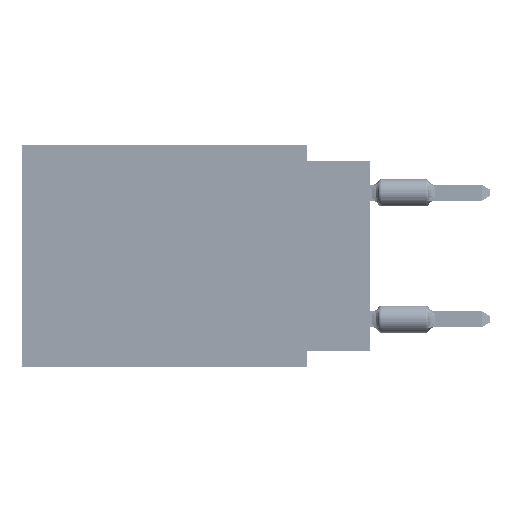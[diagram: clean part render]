
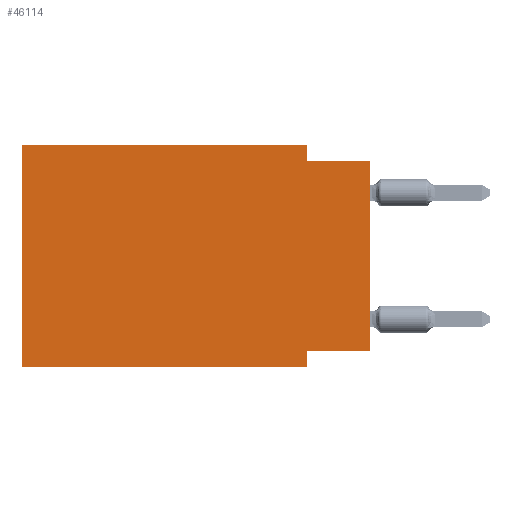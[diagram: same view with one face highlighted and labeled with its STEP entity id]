
A CAD part, left-side view. The second image highlights one B-rep face of the part: STEP entity #46114.
In plain terms, the highlighted planar face has unit normal (-1, 0, 0).
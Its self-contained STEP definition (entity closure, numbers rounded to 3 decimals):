
#430 = VECTOR ( 'NONE', #18082, 1000. ) ;
#1120 = VERTEX_POINT ( 'NONE', #33588 ) ;
#1628 = CARTESIAN_POINT ( 'NONE',  ( 0., 2.54, -8.255 ) ) ;
#1795 = DIRECTION ( 'NONE',  ( 0., 0., 1. ) ) ;
#2242 = VECTOR ( 'NONE', #56492, 1000. ) ;
#2879 = LINE ( 'NONE', #26406, #430 ) ;
#7391 = CARTESIAN_POINT ( 'NONE',  ( 0., 13.97, 0. ) ) ;
#7825 = VECTOR ( 'NONE', #49756, 1000. ) ;
#9047 = EDGE_CURVE ( 'NONE', #80433, #78331, #52441, .T. ) ;
#10928 = CARTESIAN_POINT ( 'NONE',  ( 0., 2.54, -0.635 ) ) ;
#13203 = VECTOR ( 'NONE', #89254, 1000. ) ;
#13825 = ORIENTED_EDGE ( 'NONE', *, *, #69051, .T. ) ;
#15236 = DIRECTION ( 'NONE',  ( 0., 0., 1. ) ) ;
#16129 = EDGE_CURVE ( 'NONE', #66606, #78331, #87042, .T. ) ;
#16884 = ORIENTED_EDGE ( 'NONE', *, *, #49032, .F. ) ;
#18082 = DIRECTION ( 'NONE',  ( 0., 0., -1. ) ) ;
#19843 = CARTESIAN_POINT ( 'NONE',  ( 0., 13.97, -8.89 ) ) ;
#21167 = CARTESIAN_POINT ( 'NONE',  ( 0., 13.97, 0. ) ) ;
#21896 = CARTESIAN_POINT ( 'NONE',  ( 0., 2.54, -8.89 ) ) ;
#23350 = EDGE_CURVE ( 'NONE', #74898, #35920, #65322, .T. ) ;
#25689 = EDGE_CURVE ( 'NONE', #66606, #74898, #52506, .T. ) ;
#26406 = CARTESIAN_POINT ( 'NONE',  ( 0., 2.54, 0. ) ) ;
#28214 = CARTESIAN_POINT ( 'NONE',  ( 0., 13.97, 0. ) ) ;
#28435 = VECTOR ( 'NONE', #1795, 1000. ) ;
#30696 = VECTOR ( 'NONE', #52971, 1000. ) ;
#33588 = CARTESIAN_POINT ( 'NONE',  ( 0., 0., -0.635 ) ) ;
#35566 = FACE_OUTER_BOUND ( 'NONE', #51093, .T. ) ;
#35920 = VERTEX_POINT ( 'NONE', #42188 ) ;
#36294 = CARTESIAN_POINT ( 'NONE',  ( 0., 13.97, 0. ) ) ;
#37706 = CARTESIAN_POINT ( 'NONE',  ( 0., 0., -8.255 ) ) ;
#38013 = AXIS2_PLACEMENT_3D ( 'NONE', #28214, #58125, #72854 ) ;
#39083 = CARTESIAN_POINT ( 'NONE',  ( 0., 0., 0. ) ) ;
#41335 = EDGE_CURVE ( 'NONE', #44870, #1120, #85744, .T. ) ;
#42188 = CARTESIAN_POINT ( 'NONE',  ( 0., 2.54, 0. ) ) ;
#44870 = VERTEX_POINT ( 'NONE', #10928 ) ;
#46114 = ADVANCED_FACE ( 'NONE', ( #35566 ), #50290, .F. ) ;
#46392 = CARTESIAN_POINT ( 'NONE',  ( 0., 13.97, -8.89 ) ) ;
#46993 = ORIENTED_EDGE ( 'NONE', *, *, #55658, .F. ) ;
#47496 = CARTESIAN_POINT ( 'NONE',  ( 0., 0., -0.635 ) ) ;
#49032 = EDGE_CURVE ( 'NONE', #80713, #80433, #76534, .T. ) ;
#49756 = DIRECTION ( 'NONE',  ( 0., -1., 0. ) ) ;
#50290 = PLANE ( 'NONE',  #38013 ) ;
#50908 = VECTOR ( 'NONE', #15236, 1000. ) ;
#51093 = EDGE_LOOP ( 'NONE', ( #13825, #90352, #46993, #69342, #53622, #62036, #70406, #16884 ) ) ;
#52441 = LINE ( 'NONE', #66678, #13203 ) ;
#52506 = LINE ( 'NONE', #7391, #50908 ) ;
#52971 = DIRECTION ( 'NONE',  ( 0., 1., 0. ) ) ;
#53622 = ORIENTED_EDGE ( 'NONE', *, *, #25689, .F. ) ;
#55658 = EDGE_CURVE ( 'NONE', #35920, #44870, #2879, .T. ) ;
#56492 = DIRECTION ( 'NONE',  ( 0., -1., 0. ) ) ;
#58125 = DIRECTION ( 'NONE',  ( 1., 0., 0. ) ) ;
#62036 = ORIENTED_EDGE ( 'NONE', *, *, #16129, .T. ) ;
#62291 = VECTOR ( 'NONE', #62668, 1000. ) ;
#62668 = DIRECTION ( 'NONE',  ( 0., -1., 0. ) ) ;
#65322 = LINE ( 'NONE', #21167, #2242 ) ;
#66606 = VERTEX_POINT ( 'NONE', #46392 ) ;
#66678 = CARTESIAN_POINT ( 'NONE',  ( 0., 2.54, -8.89 ) ) ;
#69051 = EDGE_CURVE ( 'NONE', #80713, #1120, #76390, .T. ) ;
#69342 = ORIENTED_EDGE ( 'NONE', *, *, #23350, .F. ) ;
#70406 = ORIENTED_EDGE ( 'NONE', *, *, #9047, .F. ) ;
#72854 = DIRECTION ( 'NONE',  ( 0., 0., -1. ) ) ;
#74898 = VERTEX_POINT ( 'NONE', #36294 ) ;
#76390 = LINE ( 'NONE', #39083, #28435 ) ;
#76534 = LINE ( 'NONE', #83889, #30696 ) ;
#78331 = VERTEX_POINT ( 'NONE', #21896 ) ;
#80433 = VERTEX_POINT ( 'NONE', #1628 ) ;
#80713 = VERTEX_POINT ( 'NONE', #37706 ) ;
#83889 = CARTESIAN_POINT ( 'NONE',  ( 0., 0., -8.255 ) ) ;
#85744 = LINE ( 'NONE', #47496, #62291 ) ;
#87042 = LINE ( 'NONE', #19843, #7825 ) ;
#89254 = DIRECTION ( 'NONE',  ( 0., 0., -1. ) ) ;
#90352 = ORIENTED_EDGE ( 'NONE', *, *, #41335, .F. ) ;
